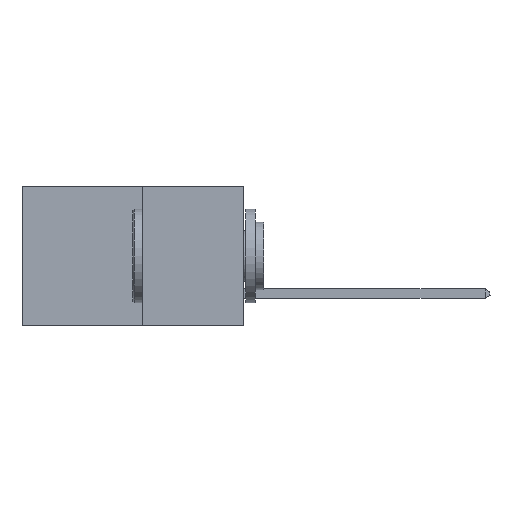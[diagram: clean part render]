
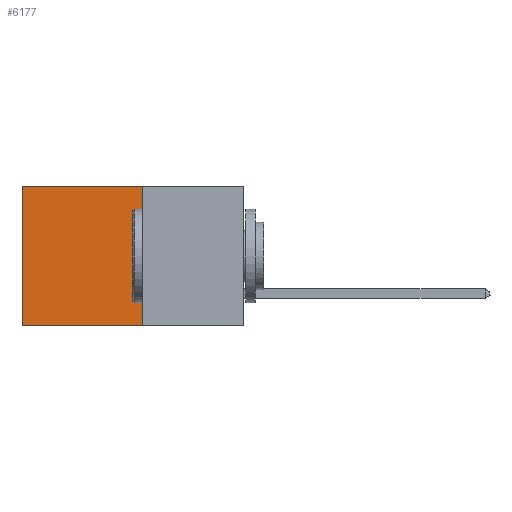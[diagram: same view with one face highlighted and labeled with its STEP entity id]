
A CAD part, left-side view. The second image highlights one B-rep face of the part: STEP entity #6177.
In plain terms, the highlighted planar face has unit normal (-1, 0, 0).
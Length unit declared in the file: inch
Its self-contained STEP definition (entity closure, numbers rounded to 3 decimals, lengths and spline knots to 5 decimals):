
#39 = VERTEX_POINT ( 'NONE', #5988 ) ;
#732 = EDGE_LOOP ( 'NONE', ( #6012, #8735, #9343, #1283 ) ) ;
#1283 = ORIENTED_EDGE ( 'NONE', *, *, #10613, .T. ) ;
#1591 = CARTESIAN_POINT ( 'NONE',  ( 0.277, 0.27, -0.37 ) ) ;
#2108 = DIRECTION ( 'NONE',  ( 0., 0., -1. ) ) ;
#2156 = VECTOR ( 'NONE', #2108, 39.37008 ) ;
#3035 = VERTEX_POINT ( 'NONE', #5203 ) ;
#3963 = DIRECTION ( 'NONE',  ( 0., 0., -1. ) ) ;
#3975 = DIRECTION ( 'NONE',  ( 1., 0., 0. ) ) ;
#3998 = PLANE ( 'NONE',  #11711 ) ;
#4093 = EDGE_CURVE ( 'NONE', #3035, #39, #10384, .T. ) ;
#4129 = CARTESIAN_POINT ( 'NONE',  ( 0.277, 0.27, -0.37 ) ) ;
#4709 = VECTOR ( 'NONE', #12346, 39.37008 ) ;
#5203 = CARTESIAN_POINT ( 'NONE',  ( 0.277, 0.59, 0. ) ) ;
#5412 = DIRECTION ( 'NONE',  ( 0., 1., 0. ) ) ;
#5988 = CARTESIAN_POINT ( 'NONE',  ( 0.277, 0.59, -0.37 ) ) ;
#6012 = ORIENTED_EDGE ( 'NONE', *, *, #4093, .T. ) ;
#6177 = ADVANCED_FACE ( 'NONE', ( #6273 ), #3998, .F. ) ;
#6273 = FACE_OUTER_BOUND ( 'NONE', #732, .T. ) ;
#6579 = EDGE_CURVE ( 'NONE', #7265, #39, #10519, .T. ) ;
#6875 = EDGE_CURVE ( 'NONE', #9617, #7265, #10358, .T. ) ;
#7265 = VERTEX_POINT ( 'NONE', #7890 ) ;
#7890 = CARTESIAN_POINT ( 'NONE',  ( 0.277, 0.27, -0.37 ) ) ;
#7987 = DIRECTION ( 'NONE',  ( 0., 1., 0. ) ) ;
#8735 = ORIENTED_EDGE ( 'NONE', *, *, #6579, .F. ) ;
#9319 = VECTOR ( 'NONE', #5412, 39.37008 ) ;
#9343 = ORIENTED_EDGE ( 'NONE', *, *, #6875, .F. ) ;
#9360 = CARTESIAN_POINT ( 'NONE',  ( 0.277, 0.27, -0.37 ) ) ;
#9617 = VERTEX_POINT ( 'NONE', #11620 ) ;
#9645 = LINE ( 'NONE', #13408, #9319 ) ;
#10358 = LINE ( 'NONE', #9360, #2156 ) ;
#10384 = LINE ( 'NONE', #11889, #4709 ) ;
#10519 = LINE ( 'NONE', #1591, #12853 ) ;
#10613 = EDGE_CURVE ( 'NONE', #9617, #3035, #9645, .T. ) ;
#11620 = CARTESIAN_POINT ( 'NONE',  ( 0.277, 0.27, 0. ) ) ;
#11711 = AXIS2_PLACEMENT_3D ( 'NONE', #4129, #3975, #3963 ) ;
#11889 = CARTESIAN_POINT ( 'NONE',  ( 0.277, 0.59, -0.37 ) ) ;
#12346 = DIRECTION ( 'NONE',  ( 0., 0., -1. ) ) ;
#12853 = VECTOR ( 'NONE', #7987, 39.37008 ) ;
#13408 = CARTESIAN_POINT ( 'NONE',  ( 0.277, 0.27, 0. ) ) ;
